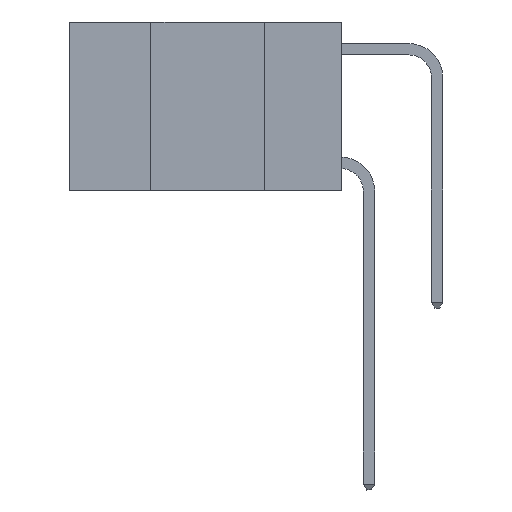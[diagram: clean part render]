
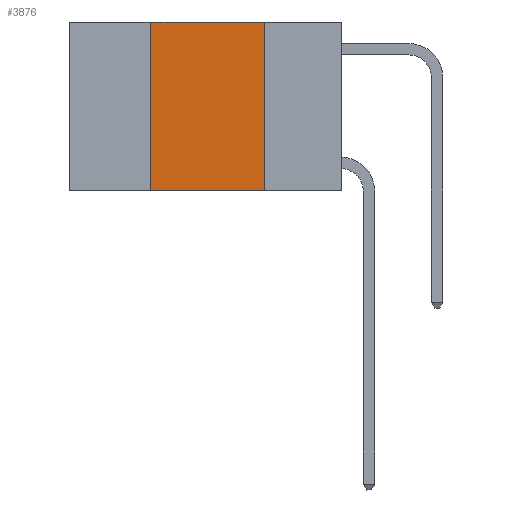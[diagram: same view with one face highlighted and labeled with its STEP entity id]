
A CAD part, left-side view. The second image highlights one B-rep face of the part: STEP entity #3876.
In plain terms, the highlighted planar face has unit normal (-1, 0, 0).
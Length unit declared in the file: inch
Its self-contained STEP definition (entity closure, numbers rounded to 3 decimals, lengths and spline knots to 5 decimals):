
#59 = EDGE_CURVE ( 'NONE', #3372, #556, #4942, .T. ) ;
#439 = CARTESIAN_POINT ( 'NONE',  ( 0., 0.17, 0. ) ) ;
#556 = VERTEX_POINT ( 'NONE', #439 ) ;
#687 = DIRECTION ( 'NONE',  ( 1., 0., 0. ) ) ;
#702 = ORIENTED_EDGE ( 'NONE', *, *, #59, .F. ) ;
#1462 = PLANE ( 'NONE',  #3974 ) ;
#1590 = CARTESIAN_POINT ( 'NONE',  ( 0., 0.6, -0.37 ) ) ;
#1653 = VECTOR ( 'NONE', #5192, 39.37008 ) ;
#1682 = ORIENTED_EDGE ( 'NONE', *, *, #7391, .F. ) ;
#2444 = CARTESIAN_POINT ( 'NONE',  ( 0., 0.17, 0. ) ) ;
#2987 = ORIENTED_EDGE ( 'NONE', *, *, #9005, .T. ) ;
#3317 = LINE ( 'NONE', #1590, #6266 ) ;
#3372 = VERTEX_POINT ( 'NONE', #7161 ) ;
#3649 = VECTOR ( 'NONE', #5556, 39.37008 ) ;
#3876 = ADVANCED_FACE ( 'NONE', ( #5375 ), #1462, .F. ) ;
#3974 = AXIS2_PLACEMENT_3D ( 'NONE', #4621, #687, #6992 ) ;
#4255 = CARTESIAN_POINT ( 'NONE',  ( 0., 0.17, -0.37 ) ) ;
#4478 = CARTESIAN_POINT ( 'NONE',  ( 0., 0.42, 0. ) ) ;
#4575 = LINE ( 'NONE', #4478, #1653 ) ;
#4621 = CARTESIAN_POINT ( 'NONE',  ( 0., 0.6, 0. ) ) ;
#4789 = EDGE_LOOP ( 'NONE', ( #8619, #702, #1682, #2987 ) ) ;
#4942 = LINE ( 'NONE', #9297, #9787 ) ;
#5192 = DIRECTION ( 'NONE',  ( 0., 0., 1. ) ) ;
#5235 = EDGE_CURVE ( 'NONE', #556, #6312, #9521, .T. ) ;
#5293 = VERTEX_POINT ( 'NONE', #6728 ) ;
#5375 = FACE_OUTER_BOUND ( 'NONE', #4789, .T. ) ;
#5556 = DIRECTION ( 'NONE',  ( 0., 0., -1. ) ) ;
#6207 = DIRECTION ( 'NONE',  ( 0., -1., 0. ) ) ;
#6266 = VECTOR ( 'NONE', #8028, 39.37008 ) ;
#6312 = VERTEX_POINT ( 'NONE', #4255 ) ;
#6728 = CARTESIAN_POINT ( 'NONE',  ( 0., 0.42, -0.37 ) ) ;
#6992 = DIRECTION ( 'NONE',  ( 0., 0., -1. ) ) ;
#7161 = CARTESIAN_POINT ( 'NONE',  ( 0., 0.42, 0. ) ) ;
#7391 = EDGE_CURVE ( 'NONE', #5293, #3372, #4575, .T. ) ;
#8028 = DIRECTION ( 'NONE',  ( 0., -1., 0. ) ) ;
#8619 = ORIENTED_EDGE ( 'NONE', *, *, #5235, .F. ) ;
#9005 = EDGE_CURVE ( 'NONE', #5293, #6312, #3317, .T. ) ;
#9297 = CARTESIAN_POINT ( 'NONE',  ( 0., 0.6, 0. ) ) ;
#9521 = LINE ( 'NONE', #2444, #3649 ) ;
#9787 = VECTOR ( 'NONE', #6207, 39.37008 ) ;
